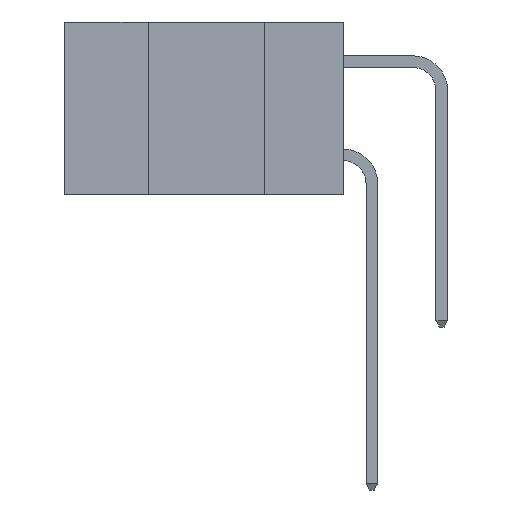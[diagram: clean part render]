
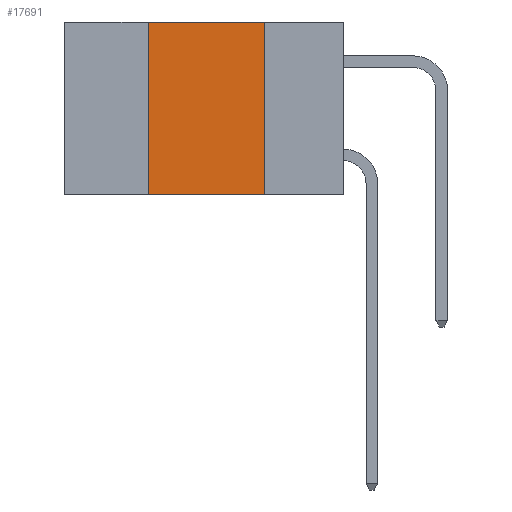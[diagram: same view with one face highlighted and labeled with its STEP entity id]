
A CAD part, left-side view. The second image highlights one B-rep face of the part: STEP entity #17691.
In plain terms, the highlighted planar face has unit normal (-1, 0, 0).
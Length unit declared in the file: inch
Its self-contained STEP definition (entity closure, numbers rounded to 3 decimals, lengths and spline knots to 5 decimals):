
#277 = VECTOR ( 'NONE', #13474, 39.37008 ) ;
#510 = VERTEX_POINT ( 'NONE', #7157 ) ;
#564 = EDGE_CURVE ( 'NONE', #7628, #510, #3683, .T. ) ;
#773 = EDGE_LOOP ( 'NONE', ( #17596, #3886, #7017, #7754 ) ) ;
#785 = VECTOR ( 'NONE', #18158, 39.37008 ) ;
#1294 = LINE ( 'NONE', #17763, #13032 ) ;
#1519 = AXIS2_PLACEMENT_3D ( 'NONE', #11228, #2050, #12732 ) ;
#2050 = DIRECTION ( 'NONE',  ( 1., 0., 0. ) ) ;
#2335 = CARTESIAN_POINT ( 'NONE',  ( 0., 0.42, 0. ) ) ;
#3637 = DIRECTION ( 'NONE',  ( 0., -1., 0. ) ) ;
#3683 = LINE ( 'NONE', #4316, #19360 ) ;
#3886 = ORIENTED_EDGE ( 'NONE', *, *, #564, .F. ) ;
#4309 = CARTESIAN_POINT ( 'NONE',  ( 0., 0.17, -0.37 ) ) ;
#4316 = CARTESIAN_POINT ( 'NONE',  ( 0., 0.6, 0. ) ) ;
#7017 = ORIENTED_EDGE ( 'NONE', *, *, #18650, .F. ) ;
#7157 = CARTESIAN_POINT ( 'NONE',  ( 0., 0.17, 0. ) ) ;
#7172 = EDGE_CURVE ( 'NONE', #9682, #15753, #1294, .T. ) ;
#7183 = DIRECTION ( 'NONE',  ( 0., -1., 0. ) ) ;
#7628 = VERTEX_POINT ( 'NONE', #2335 ) ;
#7754 = ORIENTED_EDGE ( 'NONE', *, *, #7172, .T. ) ;
#9682 = VERTEX_POINT ( 'NONE', #12218 ) ;
#10484 = FACE_OUTER_BOUND ( 'NONE', #773, .T. ) ;
#11228 = CARTESIAN_POINT ( 'NONE',  ( 0., 0.6, 0. ) ) ;
#12218 = CARTESIAN_POINT ( 'NONE',  ( 0., 0.42, -0.37 ) ) ;
#12552 = LINE ( 'NONE', #4309, #277 ) ;
#12732 = DIRECTION ( 'NONE',  ( 0., 0., -1. ) ) ;
#13032 = VECTOR ( 'NONE', #7183, 39.37008 ) ;
#13474 = DIRECTION ( 'NONE',  ( 0., 0., -1. ) ) ;
#15753 = VERTEX_POINT ( 'NONE', #18301 ) ;
#16635 = CARTESIAN_POINT ( 'NONE',  ( 0., 0.42, -0.37 ) ) ;
#17282 = PLANE ( 'NONE',  #1519 ) ;
#17586 = LINE ( 'NONE', #16635, #785 ) ;
#17596 = ORIENTED_EDGE ( 'NONE', *, *, #19126, .F. ) ;
#17691 = ADVANCED_FACE ( 'NONE', ( #10484 ), #17282, .F. ) ;
#17763 = CARTESIAN_POINT ( 'NONE',  ( 0., 0.6, -0.37 ) ) ;
#18158 = DIRECTION ( 'NONE',  ( 0., 0., 1. ) ) ;
#18301 = CARTESIAN_POINT ( 'NONE',  ( 0., 0.17, -0.37 ) ) ;
#18650 = EDGE_CURVE ( 'NONE', #9682, #7628, #17586, .T. ) ;
#19126 = EDGE_CURVE ( 'NONE', #510, #15753, #12552, .T. ) ;
#19360 = VECTOR ( 'NONE', #3637, 39.37008 ) ;
